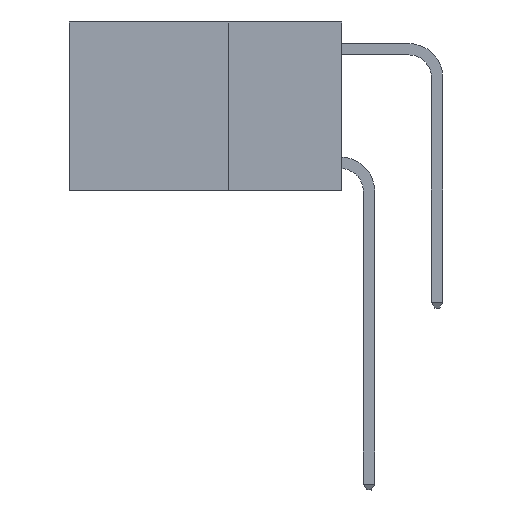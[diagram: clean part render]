
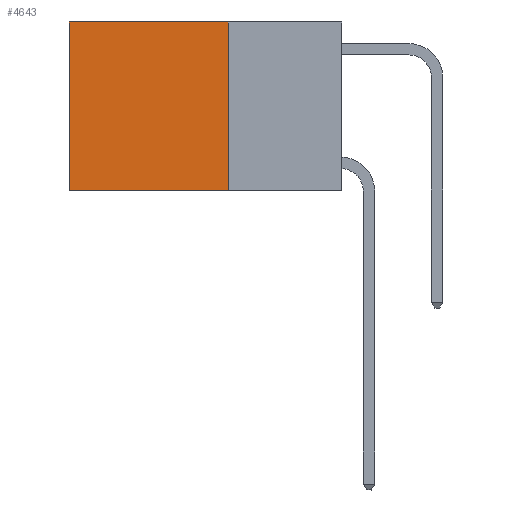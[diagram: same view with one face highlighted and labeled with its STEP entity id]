
A CAD part, left-side view. The second image highlights one B-rep face of the part: STEP entity #4643.
In plain terms, the highlighted planar face has unit normal (-1, 0, 0).
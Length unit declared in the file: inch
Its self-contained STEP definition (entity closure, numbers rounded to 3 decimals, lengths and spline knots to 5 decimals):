
#345 = EDGE_CURVE ( 'NONE', #4058, #11546, #8155, .T. ) ;
#545 = DIRECTION ( 'NONE',  ( 0., 1., 0. ) ) ;
#773 = EDGE_LOOP ( 'NONE', ( #4797, #1651, #4407, #6573 ) ) ;
#1508 = LINE ( 'NONE', #8037, #4653 ) ;
#1589 = CARTESIAN_POINT ( 'NONE',  ( 0.2625, 0.25, 0. ) ) ;
#1651 = ORIENTED_EDGE ( 'NONE', *, *, #10752, .F. ) ;
#1929 = CARTESIAN_POINT ( 'NONE',  ( 0.2625, 0.6, -0.37 ) ) ;
#2727 = EDGE_CURVE ( 'NONE', #4058, #7367, #1508, .T. ) ;
#2765 = DIRECTION ( 'NONE',  ( 1., 0., 0. ) ) ;
#3284 = FACE_OUTER_BOUND ( 'NONE', #773, .T. ) ;
#4058 = VERTEX_POINT ( 'NONE', #6099 ) ;
#4407 = ORIENTED_EDGE ( 'NONE', *, *, #345, .F. ) ;
#4643 = ADVANCED_FACE ( 'NONE', ( #3284 ), #9345, .F. ) ;
#4653 = VECTOR ( 'NONE', #5867, 39.37008 ) ;
#4797 = ORIENTED_EDGE ( 'NONE', *, *, #12879, .T. ) ;
#5795 = AXIS2_PLACEMENT_3D ( 'NONE', #1589, #2765, #10303 ) ;
#5867 = DIRECTION ( 'NONE',  ( 0., 1., 0. ) ) ;
#6099 = CARTESIAN_POINT ( 'NONE',  ( 0.2625, 0.25, 0. ) ) ;
#6531 = VERTEX_POINT ( 'NONE', #1929 ) ;
#6573 = ORIENTED_EDGE ( 'NONE', *, *, #2727, .T. ) ;
#7367 = VERTEX_POINT ( 'NONE', #10519 ) ;
#8037 = CARTESIAN_POINT ( 'NONE',  ( 0.2625, 0.25, 0. ) ) ;
#8155 = LINE ( 'NONE', #10897, #13231 ) ;
#8177 = VECTOR ( 'NONE', #8874, 39.37008 ) ;
#8308 = CARTESIAN_POINT ( 'NONE',  ( 0.2625, 0.25, -0.37 ) ) ;
#8874 = DIRECTION ( 'NONE',  ( 0., 0., -1. ) ) ;
#9000 = LINE ( 'NONE', #12254, #10977 ) ;
#9345 = PLANE ( 'NONE',  #5795 ) ;
#10303 = DIRECTION ( 'NONE',  ( 0., 0., -1. ) ) ;
#10519 = CARTESIAN_POINT ( 'NONE',  ( 0.2625, 0.6, 0. ) ) ;
#10752 = EDGE_CURVE ( 'NONE', #11546, #6531, #9000, .T. ) ;
#10897 = CARTESIAN_POINT ( 'NONE',  ( 0.2625, 0.25, 0. ) ) ;
#10977 = VECTOR ( 'NONE', #545, 39.37008 ) ;
#11546 = VERTEX_POINT ( 'NONE', #8308 ) ;
#12254 = CARTESIAN_POINT ( 'NONE',  ( 0.2625, 0.25, -0.37 ) ) ;
#12879 = EDGE_CURVE ( 'NONE', #7367, #6531, #13508, .T. ) ;
#13131 = DIRECTION ( 'NONE',  ( 0., 0., -1. ) ) ;
#13231 = VECTOR ( 'NONE', #13131, 39.37008 ) ;
#13508 = LINE ( 'NONE', #13568, #8177 ) ;
#13568 = CARTESIAN_POINT ( 'NONE',  ( 0.2625, 0.6, 0. ) ) ;
